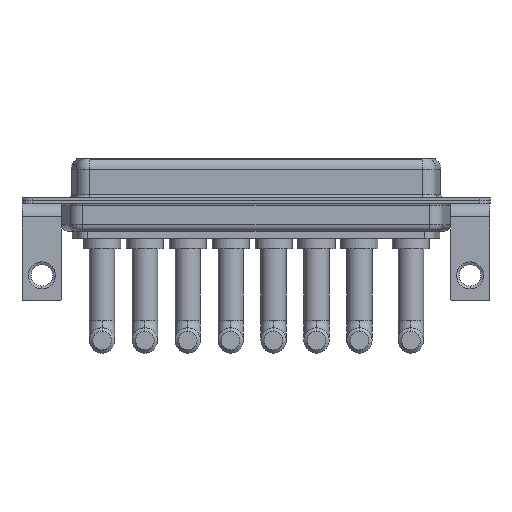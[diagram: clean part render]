
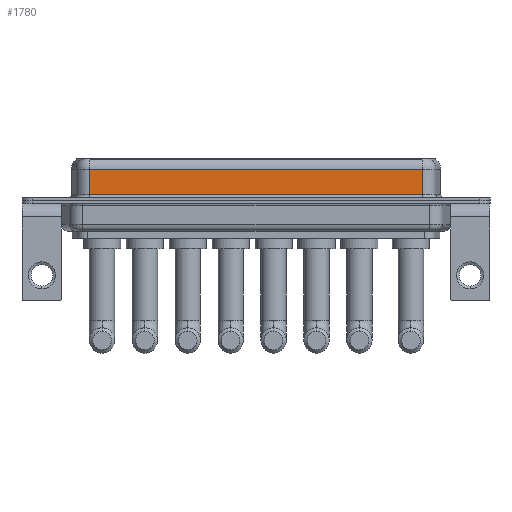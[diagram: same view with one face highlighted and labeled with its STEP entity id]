
A CAD part, front view. The second image highlights one B-rep face of the part: STEP entity #1780.
In plain terms, the highlighted planar face has unit normal (0, -1, 0).
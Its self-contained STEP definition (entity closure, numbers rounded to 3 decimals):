
#101 = CARTESIAN_POINT ( 'NONE',  ( 56.462, -3.95, 0.9 ) ) ;
#211 = EDGE_CURVE ( 'NONE', #4161, #1444, #1054, .T. ) ;
#607 = VECTOR ( 'NONE', #5236, 1000. ) ;
#895 = CARTESIAN_POINT ( 'NONE',  ( 56.462, -3.95, 4.65 ) ) ;
#1054 = LINE ( 'NONE', #5402, #3216 ) ;
#1391 = CARTESIAN_POINT ( 'NONE',  ( 56.462, -3.95, 6.4 ) ) ;
#1444 = VERTEX_POINT ( 'NONE', #6409 ) ;
#1606 = LINE ( 'NONE', #7832, #8557 ) ;
#1780 = ADVANCED_FACE ( 'NONE', ( #2456 ), #10272, .F. ) ;
#1783 = LINE ( 'NONE', #5069, #4209 ) ;
#1952 = EDGE_CURVE ( 'NONE', #13847, #4161, #6318, .T. ) ;
#2039 = VERTEX_POINT ( 'NONE', #101 ) ;
#2456 = FACE_OUTER_BOUND ( 'NONE', #8211, .T. ) ;
#3216 = VECTOR ( 'NONE', #13673, 1000. ) ;
#3810 = DIRECTION ( 'NONE',  ( 0., 1., 0. ) ) ;
#4161 = VERTEX_POINT ( 'NONE', #11385 ) ;
#4209 = VECTOR ( 'NONE', #5001, 1000. ) ;
#4214 = ORIENTED_EDGE ( 'NONE', *, *, #8643, .F. ) ;
#5001 = DIRECTION ( 'NONE',  ( 0., 0., -1. ) ) ;
#5069 = CARTESIAN_POINT ( 'NONE',  ( 56.462, -3.95, 6.4 ) ) ;
#5236 = DIRECTION ( 'NONE',  ( -1., 0., 0. ) ) ;
#5402 = CARTESIAN_POINT ( 'NONE',  ( 7.038, -3.95, 6.4 ) ) ;
#5687 = DIRECTION ( 'NONE',  ( 1., 0., 0. ) ) ;
#5749 = DIRECTION ( 'NONE',  ( 0., 0., 1. ) ) ;
#5940 = AXIS2_PLACEMENT_3D ( 'NONE', #1391, #3810, #5749 ) ;
#6318 = LINE ( 'NONE', #895, #607 ) ;
#6409 = CARTESIAN_POINT ( 'NONE',  ( 7.038, -3.95, 0.9 ) ) ;
#6609 = CARTESIAN_POINT ( 'NONE',  ( 56.462, -3.95, 4.65 ) ) ;
#7832 = CARTESIAN_POINT ( 'NONE',  ( 56.462, -3.95, 0.9 ) ) ;
#8211 = EDGE_LOOP ( 'NONE', ( #4214, #8326, #10501, #8842 ) ) ;
#8326 = ORIENTED_EDGE ( 'NONE', *, *, #1952, .T. ) ;
#8557 = VECTOR ( 'NONE', #5687, 1000. ) ;
#8643 = EDGE_CURVE ( 'NONE', #13847, #2039, #1783, .T. ) ;
#8842 = ORIENTED_EDGE ( 'NONE', *, *, #9707, .T. ) ;
#9707 = EDGE_CURVE ( 'NONE', #1444, #2039, #1606, .T. ) ;
#10272 = PLANE ( 'NONE',  #5940 ) ;
#10501 = ORIENTED_EDGE ( 'NONE', *, *, #211, .T. ) ;
#11385 = CARTESIAN_POINT ( 'NONE',  ( 7.038, -3.95, 4.65 ) ) ;
#13673 = DIRECTION ( 'NONE',  ( 0., 0., -1. ) ) ;
#13847 = VERTEX_POINT ( 'NONE', #6609 ) ;
